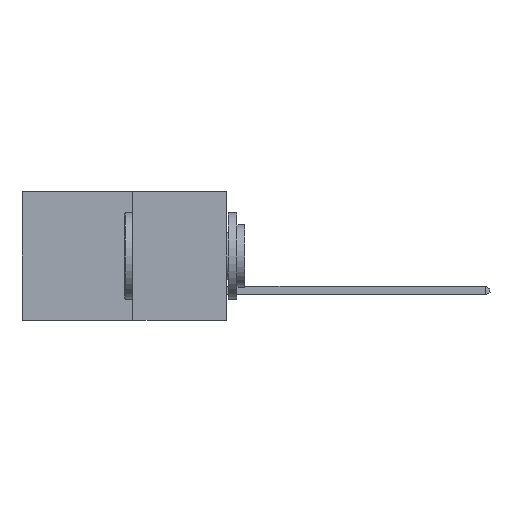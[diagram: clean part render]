
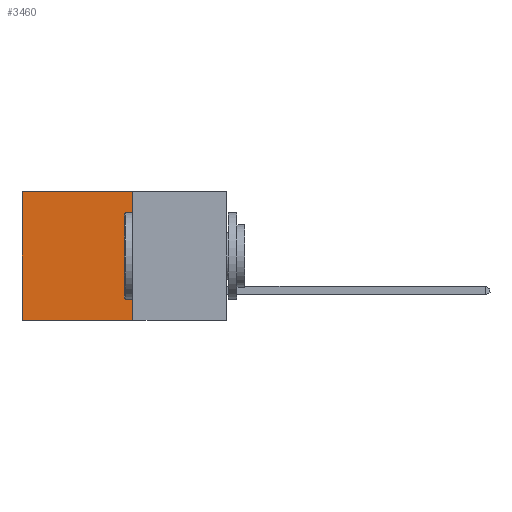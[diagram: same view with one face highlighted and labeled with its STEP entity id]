
A CAD part, left-side view. The second image highlights one B-rep face of the part: STEP entity #3460.
In plain terms, the highlighted planar face has unit normal (-1, 0, 0).
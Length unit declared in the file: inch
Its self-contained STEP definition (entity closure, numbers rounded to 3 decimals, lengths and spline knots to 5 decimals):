
#2 = CARTESIAN_POINT ( 'NONE',  ( 0.277, 0.59, -0.37 ) ) ;
#582 = EDGE_LOOP ( 'NONE', ( #5235, #1098, #4194, #4920 ) ) ;
#678 = CARTESIAN_POINT ( 'NONE',  ( 0.277, 0.27, -0.37 ) ) ;
#746 = LINE ( 'NONE', #1204, #2424 ) ;
#799 = AXIS2_PLACEMENT_3D ( 'NONE', #3158, #2443, #4346 ) ;
#941 = DIRECTION ( 'NONE',  ( 0., 0., -1. ) ) ;
#1098 = ORIENTED_EDGE ( 'NONE', *, *, #8362, .F. ) ;
#1204 = CARTESIAN_POINT ( 'NONE',  ( 0.277, 0.59, -0.37 ) ) ;
#1410 = LINE ( 'NONE', #6009, #3127 ) ;
#1603 = DIRECTION ( 'NONE',  ( 0., 1., 0. ) ) ;
#2158 = LINE ( 'NONE', #2409, #5683 ) ;
#2409 = CARTESIAN_POINT ( 'NONE',  ( 0.277, 0.27, 0. ) ) ;
#2424 = VECTOR ( 'NONE', #941, 39.37008 ) ;
#2443 = DIRECTION ( 'NONE',  ( 1., 0., 0. ) ) ;
#2872 = PLANE ( 'NONE',  #799 ) ;
#2914 = FACE_OUTER_BOUND ( 'NONE', #582, .T. ) ;
#3127 = VECTOR ( 'NONE', #5880, 39.37008 ) ;
#3154 = DIRECTION ( 'NONE',  ( 0., 1., 0. ) ) ;
#3158 = CARTESIAN_POINT ( 'NONE',  ( 0.277, 0.27, -0.37 ) ) ;
#3226 = VECTOR ( 'NONE', #1603, 39.37008 ) ;
#3304 = VERTEX_POINT ( 'NONE', #4433 ) ;
#3460 = ADVANCED_FACE ( 'NONE', ( #2914 ), #2872, .F. ) ;
#3882 = CARTESIAN_POINT ( 'NONE',  ( 0.277, 0.27, 0. ) ) ;
#4194 = ORIENTED_EDGE ( 'NONE', *, *, #5424, .F. ) ;
#4346 = DIRECTION ( 'NONE',  ( 0., 0., -1. ) ) ;
#4433 = CARTESIAN_POINT ( 'NONE',  ( 0.277, 0.59, 0. ) ) ;
#4920 = ORIENTED_EDGE ( 'NONE', *, *, #7800, .T. ) ;
#5235 = ORIENTED_EDGE ( 'NONE', *, *, #6565, .T. ) ;
#5424 = EDGE_CURVE ( 'NONE', #5521, #7346, #1410, .T. ) ;
#5521 = VERTEX_POINT ( 'NONE', #3882 ) ;
#5683 = VECTOR ( 'NONE', #3154, 39.37008 ) ;
#5880 = DIRECTION ( 'NONE',  ( 0., 0., -1. ) ) ;
#6009 = CARTESIAN_POINT ( 'NONE',  ( 0.277, 0.27, -0.37 ) ) ;
#6565 = EDGE_CURVE ( 'NONE', #3304, #6871, #746, .T. ) ;
#6871 = VERTEX_POINT ( 'NONE', #2 ) ;
#7078 = CARTESIAN_POINT ( 'NONE',  ( 0.277, 0.27, -0.37 ) ) ;
#7346 = VERTEX_POINT ( 'NONE', #678 ) ;
#7800 = EDGE_CURVE ( 'NONE', #5521, #3304, #2158, .T. ) ;
#8345 = LINE ( 'NONE', #7078, #3226 ) ;
#8362 = EDGE_CURVE ( 'NONE', #7346, #6871, #8345, .T. ) ;
